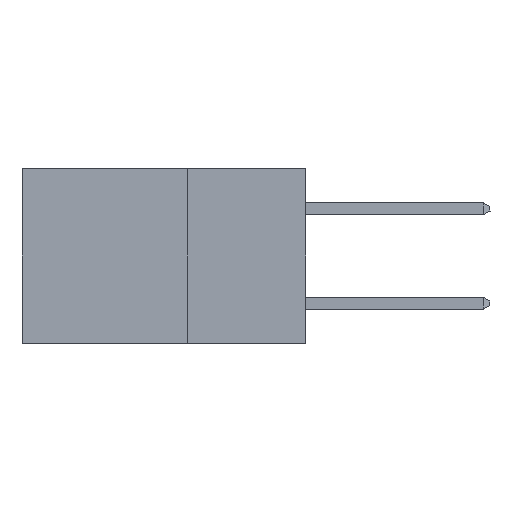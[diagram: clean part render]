
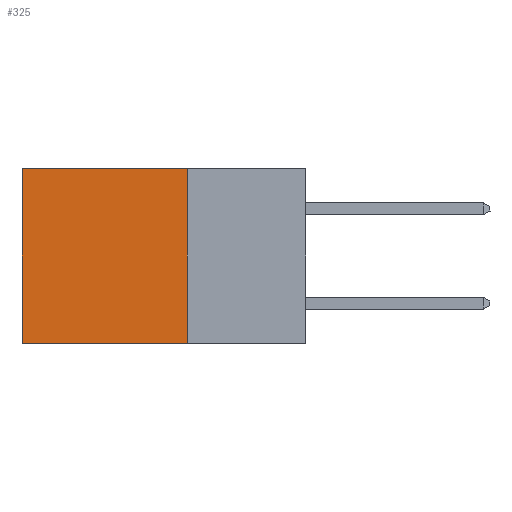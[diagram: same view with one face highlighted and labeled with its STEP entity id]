
A CAD part, left-side view. The second image highlights one B-rep face of the part: STEP entity #325.
In plain terms, the highlighted planar face has unit normal (-1, 0, 0).
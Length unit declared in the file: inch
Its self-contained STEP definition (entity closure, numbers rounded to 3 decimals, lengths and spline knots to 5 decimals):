
#196 = VECTOR ( 'NONE', #2053, 39.37008 ) ;
#325 = ADVANCED_FACE ( 'NONE', ( #8374 ), #15933, .F. ) ;
#455 = ORIENTED_EDGE ( 'NONE', *, *, #13362, .F. ) ;
#653 = CARTESIAN_POINT ( 'NONE',  ( 0.298, 0.25, 0. ) ) ;
#2053 = DIRECTION ( 'NONE',  ( 0., 0., -1. ) ) ;
#2474 = VERTEX_POINT ( 'NONE', #3190 ) ;
#2714 = EDGE_LOOP ( 'NONE', ( #12766, #455, #18502, #14019 ) ) ;
#3190 = CARTESIAN_POINT ( 'NONE',  ( 0.298, 0.25, -0.37 ) ) ;
#3705 = CARTESIAN_POINT ( 'NONE',  ( 0.298, 0.6, 0. ) ) ;
#3880 = DIRECTION ( 'NONE',  ( 1., 0., 0. ) ) ;
#6230 = VERTEX_POINT ( 'NONE', #11452 ) ;
#6547 = VECTOR ( 'NONE', #8403, 39.37008 ) ;
#8374 = FACE_OUTER_BOUND ( 'NONE', #2714, .T. ) ;
#8403 = DIRECTION ( 'NONE',  ( 0., 1., 0. ) ) ;
#8461 = VERTEX_POINT ( 'NONE', #17018 ) ;
#8501 = EDGE_CURVE ( 'NONE', #10993, #6230, #15811, .T. ) ;
#8983 = VECTOR ( 'NONE', #9945, 39.37008 ) ;
#9842 = CARTESIAN_POINT ( 'NONE',  ( 0.298, 0.25, 0. ) ) ;
#9892 = CARTESIAN_POINT ( 'NONE',  ( 0.298, 0.25, 0. ) ) ;
#9945 = DIRECTION ( 'NONE',  ( 0., 1., 0. ) ) ;
#10988 = AXIS2_PLACEMENT_3D ( 'NONE', #9892, #3880, #14498 ) ;
#10993 = VERTEX_POINT ( 'NONE', #3705 ) ;
#11126 = CARTESIAN_POINT ( 'NONE',  ( 0.298, 0.6, 0. ) ) ;
#11452 = CARTESIAN_POINT ( 'NONE',  ( 0.298, 0.6, -0.37 ) ) ;
#12766 = ORIENTED_EDGE ( 'NONE', *, *, #8501, .T. ) ;
#13042 = LINE ( 'NONE', #17490, #8983 ) ;
#13362 = EDGE_CURVE ( 'NONE', #2474, #6230, #13042, .T. ) ;
#14019 = ORIENTED_EDGE ( 'NONE', *, *, #14713, .T. ) ;
#14498 = DIRECTION ( 'NONE',  ( 0., 0., -1. ) ) ;
#14713 = EDGE_CURVE ( 'NONE', #8461, #10993, #18621, .T. ) ;
#15448 = LINE ( 'NONE', #653, #18972 ) ;
#15796 = DIRECTION ( 'NONE',  ( 0., 0., -1. ) ) ;
#15811 = LINE ( 'NONE', #11126, #196 ) ;
#15933 = PLANE ( 'NONE',  #10988 ) ;
#17018 = CARTESIAN_POINT ( 'NONE',  ( 0.298, 0.25, 0. ) ) ;
#17490 = CARTESIAN_POINT ( 'NONE',  ( 0.298, 0.25, -0.37 ) ) ;
#18502 = ORIENTED_EDGE ( 'NONE', *, *, #18949, .F. ) ;
#18621 = LINE ( 'NONE', #9842, #6547 ) ;
#18949 = EDGE_CURVE ( 'NONE', #8461, #2474, #15448, .T. ) ;
#18972 = VECTOR ( 'NONE', #15796, 39.37008 ) ;
